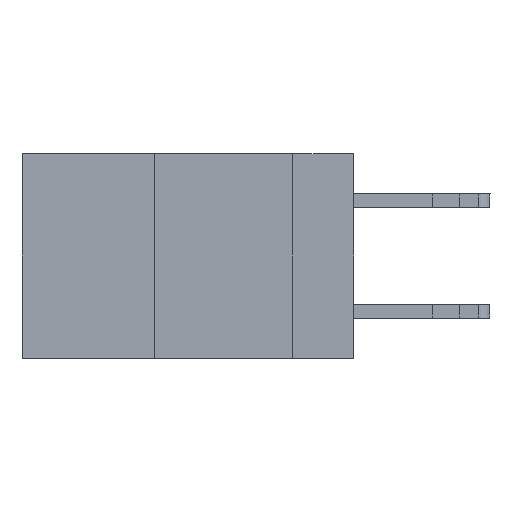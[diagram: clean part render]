
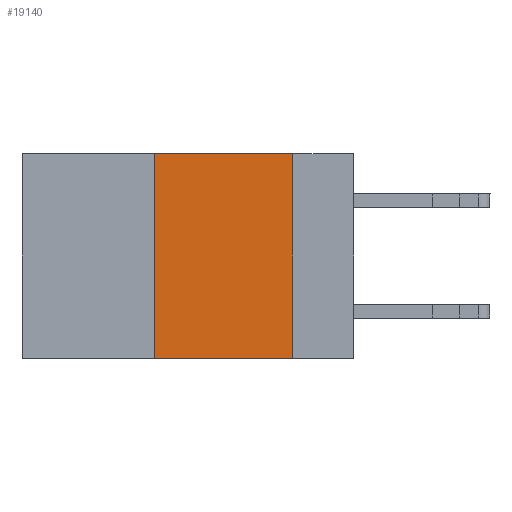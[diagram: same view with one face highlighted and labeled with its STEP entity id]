
A CAD part, left-side view. The second image highlights one B-rep face of the part: STEP entity #19140.
In plain terms, the highlighted planar face has unit normal (-1, 0, 0).
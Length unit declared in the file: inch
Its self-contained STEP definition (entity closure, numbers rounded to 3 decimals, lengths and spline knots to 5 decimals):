
#43 = DIRECTION ( 'NONE',  ( 0., -1., 0. ) ) ;
#1188 = FACE_OUTER_BOUND ( 'NONE', #4139, .T. ) ;
#1265 = LINE ( 'NONE', #16793, #14070 ) ;
#2073 = EDGE_CURVE ( 'NONE', #17771, #20747, #4238, .T. ) ;
#2195 = LINE ( 'NONE', #11867, #25014 ) ;
#2252 = ORIENTED_EDGE ( 'NONE', *, *, #6020, .F. ) ;
#2446 = DIRECTION ( 'NONE',  ( 0., 0., 1. ) ) ;
#2595 = VERTEX_POINT ( 'NONE', #8401 ) ;
#3363 = DIRECTION ( 'NONE',  ( 1., 0., 0. ) ) ;
#3790 = AXIS2_PLACEMENT_3D ( 'NONE', #13033, #3363, #12515 ) ;
#4139 = EDGE_LOOP ( 'NONE', ( #2252, #15083, #18041, #12658 ) ) ;
#4238 = LINE ( 'NONE', #13906, #4272 ) ;
#4272 = VECTOR ( 'NONE', #2446, 39.37008 ) ;
#4738 = CARTESIAN_POINT ( 'NONE',  ( 0., 0.36, 0. ) ) ;
#6020 = EDGE_CURVE ( 'NONE', #2595, #13877, #18707, .T. ) ;
#6784 = VECTOR ( 'NONE', #9300, 39.37008 ) ;
#7521 = CARTESIAN_POINT ( 'NONE',  ( 0., 0.11, 0. ) ) ;
#8401 = CARTESIAN_POINT ( 'NONE',  ( 0., 0.11, 0. ) ) ;
#9300 = DIRECTION ( 'NONE',  ( 0., 0., -1. ) ) ;
#10749 = PLANE ( 'NONE',  #3790 ) ;
#11867 = CARTESIAN_POINT ( 'NONE',  ( 0., 0.6, -0.37 ) ) ;
#12515 = DIRECTION ( 'NONE',  ( 0., 0., -1. ) ) ;
#12658 = ORIENTED_EDGE ( 'NONE', *, *, #22320, .T. ) ;
#13033 = CARTESIAN_POINT ( 'NONE',  ( 0., 0.6, 0. ) ) ;
#13659 = CARTESIAN_POINT ( 'NONE',  ( 0., 0.36, -0.37 ) ) ;
#13877 = VERTEX_POINT ( 'NONE', #23896 ) ;
#13906 = CARTESIAN_POINT ( 'NONE',  ( 0., 0.36, 0. ) ) ;
#14070 = VECTOR ( 'NONE', #24548, 39.37008 ) ;
#15083 = ORIENTED_EDGE ( 'NONE', *, *, #22655, .F. ) ;
#16793 = CARTESIAN_POINT ( 'NONE',  ( 0., 0.6, 0. ) ) ;
#17771 = VERTEX_POINT ( 'NONE', #13659 ) ;
#18041 = ORIENTED_EDGE ( 'NONE', *, *, #2073, .F. ) ;
#18707 = LINE ( 'NONE', #7521, #6784 ) ;
#19140 = ADVANCED_FACE ( 'NONE', ( #1188 ), #10749, .F. ) ;
#20747 = VERTEX_POINT ( 'NONE', #4738 ) ;
#22320 = EDGE_CURVE ( 'NONE', #17771, #13877, #2195, .T. ) ;
#22655 = EDGE_CURVE ( 'NONE', #20747, #2595, #1265, .T. ) ;
#23896 = CARTESIAN_POINT ( 'NONE',  ( 0., 0.11, -0.37 ) ) ;
#24548 = DIRECTION ( 'NONE',  ( 0., -1., 0. ) ) ;
#25014 = VECTOR ( 'NONE', #43, 39.37008 ) ;
